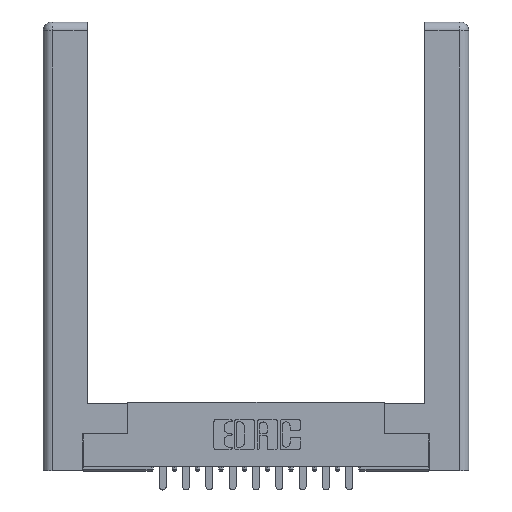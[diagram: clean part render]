
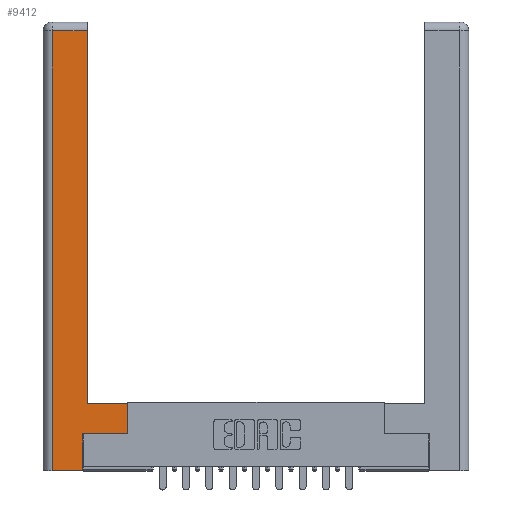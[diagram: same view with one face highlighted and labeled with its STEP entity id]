
A CAD part, top view. The second image highlights one B-rep face of the part: STEP entity #9412.
In plain terms, the highlighted planar face has unit normal (0, 0, 1).
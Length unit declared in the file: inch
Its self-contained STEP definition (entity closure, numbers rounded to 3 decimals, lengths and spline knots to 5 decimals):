
#562 = VERTEX_POINT ( 'NONE', #15640 ) ;
#689 = VECTOR ( 'NONE', #10849, 39.37008 ) ;
#901 = CARTESIAN_POINT ( 'NONE',  ( 0.0615, 0., 0. ) ) ;
#926 = LINE ( 'NONE', #10572, #13872 ) ;
#945 = ORIENTED_EDGE ( 'NONE', *, *, #6906, .T. ) ;
#1721 = EDGE_LOOP ( 'NONE', ( #14838, #6163, #945, #4385, #2962, #6450, #11392, #8672 ) ) ;
#1947 = VERTEX_POINT ( 'NONE', #8750 ) ;
#2087 = DIRECTION ( 'NONE',  ( 0., 0., -1. ) ) ;
#2681 = CARTESIAN_POINT ( 'NONE',  ( 0.295, 0.45, 0. ) ) ;
#2868 = EDGE_CURVE ( 'NONE', #13824, #5476, #12596, .T. ) ;
#2962 = ORIENTED_EDGE ( 'NONE', *, *, #12509, .T. ) ;
#3023 = VECTOR ( 'NONE', #5849, 39.37008 ) ;
#3450 = VECTOR ( 'NONE', #5519, 39.37008 ) ;
#3818 = LINE ( 'NONE', #12018, #3023 ) ;
#4385 = ORIENTED_EDGE ( 'NONE', *, *, #13214, .T. ) ;
#5047 = CARTESIAN_POINT ( 'NONE',  ( 0.295, 0.45, 0. ) ) ;
#5157 = EDGE_CURVE ( 'NONE', #1947, #12379, #926, .T. ) ;
#5239 = CARTESIAN_POINT ( 'NONE',  ( 0.0615, 2.94, 0. ) ) ;
#5476 = VERTEX_POINT ( 'NONE', #5047 ) ;
#5519 = DIRECTION ( 'NONE',  ( 0., 1., 0. ) ) ;
#5564 = DIRECTION ( 'NONE',  ( 0., -1., 0. ) ) ;
#5849 = DIRECTION ( 'NONE',  ( 0., 1., 0. ) ) ;
#6132 = LINE ( 'NONE', #14040, #16174 ) ;
#6163 = ORIENTED_EDGE ( 'NONE', *, *, #7622, .T. ) ;
#6450 = ORIENTED_EDGE ( 'NONE', *, *, #5157, .T. ) ;
#6777 = CARTESIAN_POINT ( 'NONE',  ( 0.295, 2.94, 0. ) ) ;
#6906 = EDGE_CURVE ( 'NONE', #9885, #6967, #15412, .T. ) ;
#6967 = VERTEX_POINT ( 'NONE', #901 ) ;
#7092 = VECTOR ( 'NONE', #11630, 39.37008 ) ;
#7622 = EDGE_CURVE ( 'NONE', #9775, #9885, #13830, .T. ) ;
#7844 = DIRECTION ( 'NONE',  ( -1., 0., 0. ) ) ;
#8262 = CARTESIAN_POINT ( 'NONE',  ( 0.295, 3., 0. ) ) ;
#8672 = ORIENTED_EDGE ( 'NONE', *, *, #2868, .T. ) ;
#8750 = CARTESIAN_POINT ( 'NONE',  ( 0.265, 0.245, 0. ) ) ;
#9304 = CARTESIAN_POINT ( 'NONE',  ( 0.0615, 0., 0. ) ) ;
#9412 = ADVANCED_FACE ( 'NONE', ( #12808 ), #12093, .F. ) ;
#9775 = VERTEX_POINT ( 'NONE', #6777 ) ;
#9885 = VERTEX_POINT ( 'NONE', #5239 ) ;
#10111 = VECTOR ( 'NONE', #5564, 39.37008 ) ;
#10140 = LINE ( 'NONE', #14225, #3450 ) ;
#10190 = AXIS2_PLACEMENT_3D ( 'NONE', #14704, #2087, #10980 ) ;
#10508 = VECTOR ( 'NONE', #7844, 39.37008 ) ;
#10552 = CARTESIAN_POINT ( 'NONE',  ( 0.0615, 2.94, 0. ) ) ;
#10572 = CARTESIAN_POINT ( 'NONE',  ( 0.565, 0.245, 0. ) ) ;
#10849 = DIRECTION ( 'NONE',  ( 0., 1., 0. ) ) ;
#10877 = LINE ( 'NONE', #8262, #689 ) ;
#10980 = DIRECTION ( 'NONE',  ( -1., 0., 0. ) ) ;
#11392 = ORIENTED_EDGE ( 'NONE', *, *, #11787, .T. ) ;
#11630 = DIRECTION ( 'NONE',  ( -1., 0., 0. ) ) ;
#11787 = EDGE_CURVE ( 'NONE', #12379, #13824, #10140, .T. ) ;
#12018 = CARTESIAN_POINT ( 'NONE',  ( 0.265, 0.245, 0. ) ) ;
#12093 = PLANE ( 'NONE',  #10190 ) ;
#12379 = VERTEX_POINT ( 'NONE', #14302 ) ;
#12452 = CARTESIAN_POINT ( 'NONE',  ( 0.565, 0.45, 0. ) ) ;
#12509 = EDGE_CURVE ( 'NONE', #562, #1947, #3818, .T. ) ;
#12596 = LINE ( 'NONE', #2681, #7092 ) ;
#12611 = EDGE_CURVE ( 'NONE', #5476, #9775, #10877, .T. ) ;
#12808 = FACE_OUTER_BOUND ( 'NONE', #1721, .T. ) ;
#13214 = EDGE_CURVE ( 'NONE', #6967, #562, #6132, .T. ) ;
#13824 = VERTEX_POINT ( 'NONE', #12452 ) ;
#13830 = LINE ( 'NONE', #10552, #10508 ) ;
#13872 = VECTOR ( 'NONE', #14385, 39.37008 ) ;
#14040 = CARTESIAN_POINT ( 'NONE',  ( 0.265, 0., 0. ) ) ;
#14225 = CARTESIAN_POINT ( 'NONE',  ( 0.565, 0.45, 0. ) ) ;
#14302 = CARTESIAN_POINT ( 'NONE',  ( 0.565, 0.245, 0. ) ) ;
#14385 = DIRECTION ( 'NONE',  ( 1., 0., 0. ) ) ;
#14704 = CARTESIAN_POINT ( 'NONE',  ( 0., 0., 0. ) ) ;
#14838 = ORIENTED_EDGE ( 'NONE', *, *, #12611, .T. ) ;
#15319 = DIRECTION ( 'NONE',  ( 1., 0., 0. ) ) ;
#15412 = LINE ( 'NONE', #9304, #10111 ) ;
#15640 = CARTESIAN_POINT ( 'NONE',  ( 0.265, 0., 0. ) ) ;
#16174 = VECTOR ( 'NONE', #15319, 39.37008 ) ;
